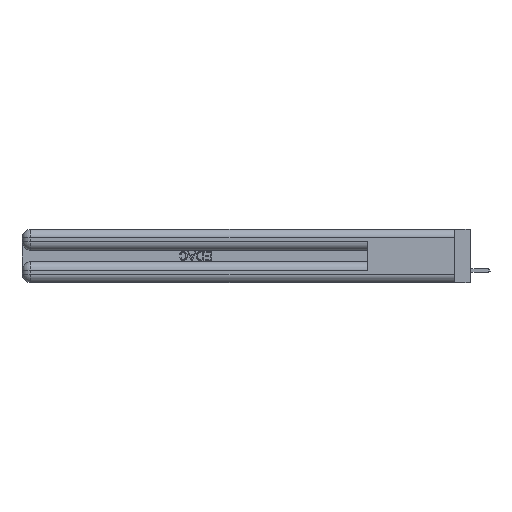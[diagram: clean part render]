
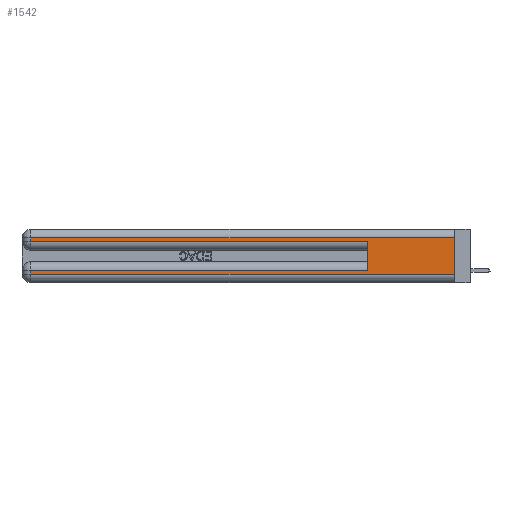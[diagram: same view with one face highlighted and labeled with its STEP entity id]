
A CAD part, left-side view. The second image highlights one B-rep face of the part: STEP entity #1542.
In plain terms, the highlighted planar face has unit normal (-1, 0, 0).
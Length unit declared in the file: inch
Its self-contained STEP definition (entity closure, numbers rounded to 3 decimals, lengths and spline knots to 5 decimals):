
#314 = DIRECTION ( 'NONE',  ( 1., 0., 0. ) ) ;
#490 = CARTESIAN_POINT ( 'NONE',  ( 0., 0., 0.31 ) ) ;
#1023 = LINE ( 'NONE', #490, #40924 ) ;
#1542 = ADVANCED_FACE ( 'NONE', ( #45726 ), #27304, .F. ) ;
#1914 = VECTOR ( 'NONE', #20317, 39.37008 ) ;
#1985 = VECTOR ( 'NONE', #39846, 39.37008 ) ;
#3593 = EDGE_CURVE ( 'NONE', #38551, #24467, #19076, .T. ) ;
#3863 = CARTESIAN_POINT ( 'NONE',  ( 0., 2.94, 0.31 ) ) ;
#4232 = DIRECTION ( 'NONE',  ( 0., 0., -1. ) ) ;
#6481 = CARTESIAN_POINT ( 'NONE',  ( 0., 0., 0.37 ) ) ;
#7503 = ORIENTED_EDGE ( 'NONE', *, *, #48212, .T. ) ;
#8371 = CARTESIAN_POINT ( 'NONE',  ( 0., 0., 0.06 ) ) ;
#8504 = VERTEX_POINT ( 'NONE', #22828 ) ;
#8738 = CARTESIAN_POINT ( 'NONE',  ( 0., 2.94, 0.37 ) ) ;
#9971 = CARTESIAN_POINT ( 'NONE',  ( 0., 0.6, 0.085 ) ) ;
#12292 = DIRECTION ( 'NONE',  ( 0., 0., -1. ) ) ;
#13286 = CARTESIAN_POINT ( 'NONE',  ( 0., 2.94, 0.085 ) ) ;
#16183 = VECTOR ( 'NONE', #43414, 39.37008 ) ;
#17148 = VERTEX_POINT ( 'NONE', #35795 ) ;
#19076 = LINE ( 'NONE', #36493, #32273 ) ;
#20317 = DIRECTION ( 'NONE',  ( 0., 0., 1. ) ) ;
#22397 = VECTOR ( 'NONE', #24594, 39.37008 ) ;
#22828 = CARTESIAN_POINT ( 'NONE',  ( 0., 0., 0.31 ) ) ;
#23301 = ORIENTED_EDGE ( 'NONE', *, *, #48216, .T. ) ;
#24220 = ORIENTED_EDGE ( 'NONE', *, *, #34427, .T. ) ;
#24467 = VERTEX_POINT ( 'NONE', #8371 ) ;
#24594 = DIRECTION ( 'NONE',  ( 0., 0., -1. ) ) ;
#25102 = AXIS2_PLACEMENT_3D ( 'NONE', #29292, #314, #4232 ) ;
#26309 = CARTESIAN_POINT ( 'NONE',  ( 0., 2.94, 0.06 ) ) ;
#26914 = EDGE_CURVE ( 'NONE', #36387, #37644, #33974, .T. ) ;
#27304 = PLANE ( 'NONE',  #25102 ) ;
#27782 = LINE ( 'NONE', #6481, #22397 ) ;
#28227 = EDGE_CURVE ( 'NONE', #8504, #24467, #27782, .T. ) ;
#28442 = DIRECTION ( 'NONE',  ( 0., -1., 0. ) ) ;
#29102 = ORIENTED_EDGE ( 'NONE', *, *, #43814, .T. ) ;
#29292 = CARTESIAN_POINT ( 'NONE',  ( 0., 0., 0.37 ) ) ;
#29868 = LINE ( 'NONE', #41299, #44917 ) ;
#29967 = EDGE_CURVE ( 'NONE', #8504, #48043, #1023, .T. ) ;
#31960 = ORIENTED_EDGE ( 'NONE', *, *, #28227, .F. ) ;
#32273 = VECTOR ( 'NONE', #28442, 39.37008 ) ;
#33068 = LINE ( 'NONE', #8738, #49315 ) ;
#33974 = LINE ( 'NONE', #43338, #1914 ) ;
#34427 = EDGE_CURVE ( 'NONE', #48043, #17148, #43026, .T. ) ;
#34781 = DIRECTION ( 'NONE',  ( 0., 1., 0. ) ) ;
#35625 = CARTESIAN_POINT ( 'NONE',  ( 0., 2.94, 0.37 ) ) ;
#35795 = CARTESIAN_POINT ( 'NONE',  ( 0., 2.94, 0.285 ) ) ;
#35996 = ORIENTED_EDGE ( 'NONE', *, *, #26914, .F. ) ;
#36387 = VERTEX_POINT ( 'NONE', #9971 ) ;
#36493 = CARTESIAN_POINT ( 'NONE',  ( 0., 0., 0.06 ) ) ;
#37644 = VERTEX_POINT ( 'NONE', #44195 ) ;
#38407 = EDGE_LOOP ( 'NONE', ( #31960, #39322, #24220, #29102, #35996, #23301, #7503, #41833 ) ) ;
#38551 = VERTEX_POINT ( 'NONE', #26309 ) ;
#39220 = CARTESIAN_POINT ( 'NONE',  ( 0., 0., 0.085 ) ) ;
#39322 = ORIENTED_EDGE ( 'NONE', *, *, #29967, .T. ) ;
#39846 = DIRECTION ( 'NONE',  ( 0., 0., -1. ) ) ;
#40924 = VECTOR ( 'NONE', #34781, 39.37008 ) ;
#41299 = CARTESIAN_POINT ( 'NONE',  ( 0., 0., 0.285 ) ) ;
#41833 = ORIENTED_EDGE ( 'NONE', *, *, #3593, .T. ) ;
#42591 = VERTEX_POINT ( 'NONE', #13286 ) ;
#43026 = LINE ( 'NONE', #35625, #1985 ) ;
#43338 = CARTESIAN_POINT ( 'NONE',  ( 0., 0.6, 0.145 ) ) ;
#43414 = DIRECTION ( 'NONE',  ( 0., 1., 0. ) ) ;
#43814 = EDGE_CURVE ( 'NONE', #17148, #37644, #29868, .T. ) ;
#44195 = CARTESIAN_POINT ( 'NONE',  ( 0., 0.6, 0.285 ) ) ;
#44491 = LINE ( 'NONE', #39220, #16183 ) ;
#44917 = VECTOR ( 'NONE', #44984, 39.37008 ) ;
#44984 = DIRECTION ( 'NONE',  ( 0., -1., 0. ) ) ;
#45726 = FACE_OUTER_BOUND ( 'NONE', #38407, .T. ) ;
#48043 = VERTEX_POINT ( 'NONE', #3863 ) ;
#48212 = EDGE_CURVE ( 'NONE', #42591, #38551, #33068, .T. ) ;
#48216 = EDGE_CURVE ( 'NONE', #36387, #42591, #44491, .T. ) ;
#49315 = VECTOR ( 'NONE', #12292, 39.37008 ) ;
